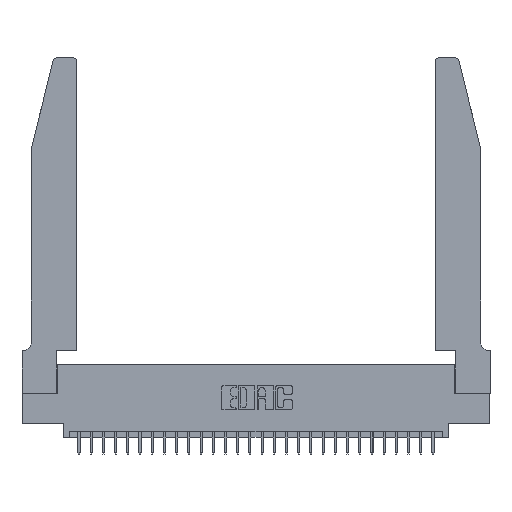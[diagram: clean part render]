
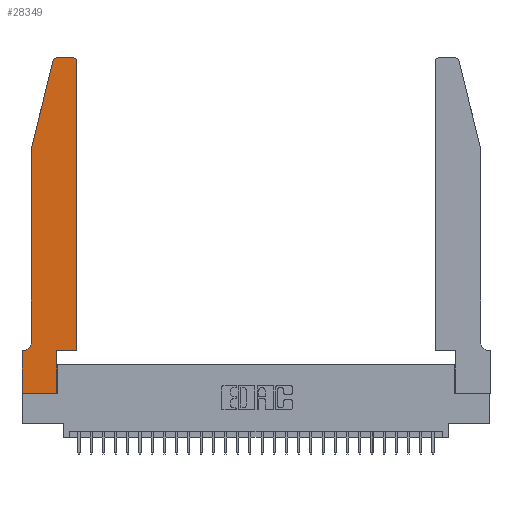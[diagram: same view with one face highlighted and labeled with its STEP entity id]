
A CAD part, top view. The second image highlights one B-rep face of the part: STEP entity #28349.
In plain terms, the highlighted planar face has unit normal (0, 0, 1).
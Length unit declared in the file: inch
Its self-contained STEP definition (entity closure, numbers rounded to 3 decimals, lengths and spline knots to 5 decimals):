
#511 = CARTESIAN_POINT ( 'NONE',  ( 0.4505, 0.35, 0.37 ) ) ;
#808 = DIRECTION ( 'NONE',  ( 0., 1., 0. ) ) ;
#1202 = VERTEX_POINT ( 'NONE', #1916 ) ;
#1714 = PLANE ( 'NONE',  #20781 ) ;
#1734 = EDGE_CURVE ( 'NONE', #19250, #18853, #19100, .T. ) ;
#1916 = CARTESIAN_POINT ( 'NONE',  ( 0.0055, 0.35, 0.37 ) ) ;
#2082 = DIRECTION ( 'NONE',  ( 1., 0., 0. ) ) ;
#3584 = EDGE_CURVE ( 'NONE', #25311, #20035, #5546, .T. ) ;
#3900 = DIRECTION ( 'NONE',  ( -1., 0., 0. ) ) ;
#3941 = ORIENTED_EDGE ( 'NONE', *, *, #3584, .T. ) ;
#4297 = VERTEX_POINT ( 'NONE', #14573 ) ;
#5184 = FACE_OUTER_BOUND ( 'NONE', #6922, .T. ) ;
#5421 = ORIENTED_EDGE ( 'NONE', *, *, #14691, .T. ) ;
#5546 = LINE ( 'NONE', #15280, #18448 ) ;
#5779 = CARTESIAN_POINT ( 'NONE',  ( 0., 0.35, 0.37 ) ) ;
#5805 = EDGE_CURVE ( 'NONE', #5814, #4297, #12390, .T. ) ;
#5814 = VERTEX_POINT ( 'NONE', #26325 ) ;
#6595 = EDGE_CURVE ( 'NONE', #7052, #19220, #14889, .T. ) ;
#6623 = DIRECTION ( 'NONE',  ( 0., 0., -1. ) ) ;
#6922 = EDGE_LOOP ( 'NONE', ( #9441, #5421, #13856, #26108, #14273, #10311, #23868, #27422, #19439, #3941, #14267, #21659 ) ) ;
#7052 = VERTEX_POINT ( 'NONE', #27055 ) ;
#7082 = DIRECTION ( 'NONE',  ( -1., 0., 0. ) ) ;
#7331 = CARTESIAN_POINT ( 'NONE',  ( 0., 0.35, 0.37 ) ) ;
#7473 = CARTESIAN_POINT ( 'NONE',  ( 0.0755, 0.35, 0.37 ) ) ;
#7668 = EDGE_CURVE ( 'NONE', #20035, #19250, #26473, .T. ) ;
#8069 = VERTEX_POINT ( 'NONE', #10413 ) ;
#8354 = VECTOR ( 'NONE', #12623, 39.37008 ) ;
#8635 = CIRCLE ( 'NONE', #11567, 0.03 ) ;
#8737 = LINE ( 'NONE', #18041, #10503 ) ;
#8981 = DIRECTION ( 'NONE',  ( 0., 1., 0. ) ) ;
#9057 = VERTEX_POINT ( 'NONE', #15525 ) ;
#9163 = CARTESIAN_POINT ( 'NONE',  ( 0., 0., 0.37 ) ) ;
#9359 = VECTOR ( 'NONE', #7082, 39.37008 ) ;
#9441 = ORIENTED_EDGE ( 'NONE', *, *, #23855, .T. ) ;
#10311 = ORIENTED_EDGE ( 'NONE', *, *, #15180, .T. ) ;
#10413 = CARTESIAN_POINT ( 'NONE',  ( 0.284, 2.75, 0.37 ) ) ;
#10503 = VECTOR ( 'NONE', #27413, 39.37008 ) ;
#11185 = VERTEX_POINT ( 'NONE', #7331 ) ;
#11567 = AXIS2_PLACEMENT_3D ( 'NONE', #22961, #17888, #2082 ) ;
#12345 = VECTOR ( 'NONE', #23370, 39.37008 ) ;
#12390 = LINE ( 'NONE', #19707, #20549 ) ;
#12559 = DIRECTION ( 'NONE',  ( 1., 0., 0. ) ) ;
#12623 = DIRECTION ( 'NONE',  ( -0.239, -0.971, 0. ) ) ;
#12715 = VECTOR ( 'NONE', #808, 39.37008 ) ;
#12988 = EDGE_CURVE ( 'NONE', #19220, #9057, #8737, .T. ) ;
#13579 = AXIS2_PLACEMENT_3D ( 'NONE', #15768, #6623, #3900 ) ;
#13700 = CARTESIAN_POINT ( 'NONE',  ( 0.4205, 2.72, 0.37 ) ) ;
#13847 = DIRECTION ( 'NONE',  ( 0., 0., 1. ) ) ;
#13856 = ORIENTED_EDGE ( 'NONE', *, *, #6595, .T. ) ;
#14267 = ORIENTED_EDGE ( 'NONE', *, *, #7668, .T. ) ;
#14273 = ORIENTED_EDGE ( 'NONE', *, *, #17941, .T. ) ;
#14573 = CARTESIAN_POINT ( 'NONE',  ( 0.2865, 0., 0.37 ) ) ;
#14691 = EDGE_CURVE ( 'NONE', #8069, #7052, #8635, .T. ) ;
#14889 = LINE ( 'NONE', #24259, #8354 ) ;
#15180 = EDGE_CURVE ( 'NONE', #1202, #11185, #25980, .T. ) ;
#15280 = CARTESIAN_POINT ( 'NONE',  ( 0.4505, 0.35, 0.37 ) ) ;
#15504 = CIRCLE ( 'NONE', #13579, 0.07 ) ;
#15525 = CARTESIAN_POINT ( 'NONE',  ( 0.0755, 0.42, 0.37 ) ) ;
#15768 = CARTESIAN_POINT ( 'NONE',  ( 0.0055, 0.42, 0.37 ) ) ;
#15909 = CARTESIAN_POINT ( 'NONE',  ( 0.2865, 0.35, 0.37 ) ) ;
#16766 = DIRECTION ( 'NONE',  ( -1., 0., 0. ) ) ;
#17430 = VECTOR ( 'NONE', #16766, 39.37008 ) ;
#17510 = DIRECTION ( 'NONE',  ( 0., 0., 1. ) ) ;
#17888 = DIRECTION ( 'NONE',  ( 0., 0., 1. ) ) ;
#17941 = EDGE_CURVE ( 'NONE', #9057, #1202, #15504, .T. ) ;
#17979 = CARTESIAN_POINT ( 'NONE',  ( 0.4505, 0.35, 0.37 ) ) ;
#18041 = CARTESIAN_POINT ( 'NONE',  ( 0.0755, 2., 0.37 ) ) ;
#18448 = VECTOR ( 'NONE', #12559, 39.37008 ) ;
#18853 = VERTEX_POINT ( 'NONE', #26126 ) ;
#18958 = EDGE_CURVE ( 'NONE', #4297, #25311, #24127, .T. ) ;
#19100 = CIRCLE ( 'NONE', #21571, 0.03 ) ;
#19220 = VERTEX_POINT ( 'NONE', #29487 ) ;
#19250 = VERTEX_POINT ( 'NONE', #27185 ) ;
#19439 = ORIENTED_EDGE ( 'NONE', *, *, #18958, .T. ) ;
#19707 = CARTESIAN_POINT ( 'NONE',  ( 0., 0., 0.37 ) ) ;
#20035 = VERTEX_POINT ( 'NONE', #511 ) ;
#20549 = VECTOR ( 'NONE', #21720, 39.37008 ) ;
#20781 = AXIS2_PLACEMENT_3D ( 'NONE', #5779, #17510, #24589 ) ;
#20977 = CARTESIAN_POINT ( 'NONE',  ( 0.2605, 2.75, 0.37 ) ) ;
#21571 = AXIS2_PLACEMENT_3D ( 'NONE', #13700, #13847, #23199 ) ;
#21659 = ORIENTED_EDGE ( 'NONE', *, *, #1734, .T. ) ;
#21720 = DIRECTION ( 'NONE',  ( 1., 0., 0. ) ) ;
#21821 = CARTESIAN_POINT ( 'NONE',  ( 0.2865, 0.35, 0.37 ) ) ;
#22601 = VECTOR ( 'NONE', #8981, 39.37008 ) ;
#22961 = CARTESIAN_POINT ( 'NONE',  ( 0.284, 2.72, 0.37 ) ) ;
#23199 = DIRECTION ( 'NONE',  ( 1., 0., 0. ) ) ;
#23370 = DIRECTION ( 'NONE',  ( 0., -1., 0. ) ) ;
#23855 = EDGE_CURVE ( 'NONE', #18853, #8069, #27894, .T. ) ;
#23868 = ORIENTED_EDGE ( 'NONE', *, *, #25510, .T. ) ;
#24127 = LINE ( 'NONE', #21821, #12715 ) ;
#24259 = CARTESIAN_POINT ( 'NONE',  ( 0.0755, 2., 0.37 ) ) ;
#24589 = DIRECTION ( 'NONE',  ( 1., 0., 0. ) ) ;
#25311 = VERTEX_POINT ( 'NONE', #15909 ) ;
#25510 = EDGE_CURVE ( 'NONE', #11185, #5814, #26768, .T. ) ;
#25980 = LINE ( 'NONE', #7473, #17430 ) ;
#26108 = ORIENTED_EDGE ( 'NONE', *, *, #12988, .T. ) ;
#26126 = CARTESIAN_POINT ( 'NONE',  ( 0.4205, 2.75, 0.37 ) ) ;
#26325 = CARTESIAN_POINT ( 'NONE',  ( 0., 0., 0.37 ) ) ;
#26473 = LINE ( 'NONE', #17979, #22601 ) ;
#26768 = LINE ( 'NONE', #9163, #12345 ) ;
#27055 = CARTESIAN_POINT ( 'NONE',  ( 0.25487, 2.72718, 0.37 ) ) ;
#27185 = CARTESIAN_POINT ( 'NONE',  ( 0.4505, 2.72, 0.37 ) ) ;
#27413 = DIRECTION ( 'NONE',  ( 0., -1., 0. ) ) ;
#27422 = ORIENTED_EDGE ( 'NONE', *, *, #5805, .T. ) ;
#27894 = LINE ( 'NONE', #20977, #9359 ) ;
#28349 = ADVANCED_FACE ( 'NONE', ( #5184 ), #1714, .T. ) ;
#29487 = CARTESIAN_POINT ( 'NONE',  ( 0.0755, 2., 0.37 ) ) ;
